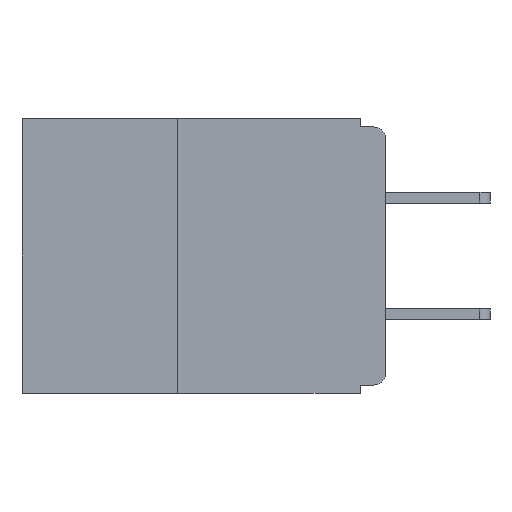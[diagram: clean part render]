
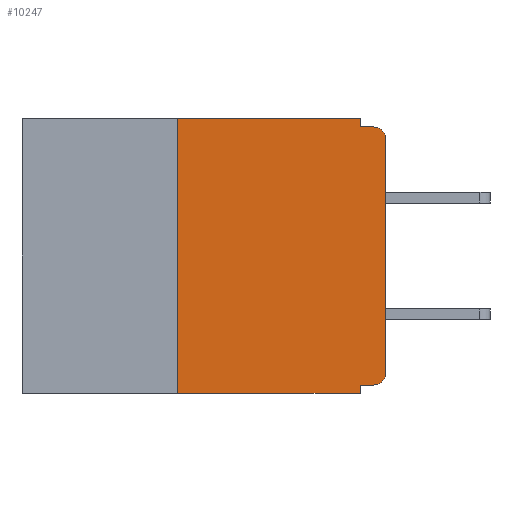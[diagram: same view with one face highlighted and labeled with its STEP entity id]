
A CAD part, left-side view. The second image highlights one B-rep face of the part: STEP entity #10247.
In plain terms, the highlighted planar face has unit normal (-1, 0, 0).
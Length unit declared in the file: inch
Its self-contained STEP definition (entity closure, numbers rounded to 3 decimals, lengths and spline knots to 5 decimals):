
#102 = PLANE ( 'NONE',  #8327 ) ;
#334 = LINE ( 'NONE', #4400, #4716 ) ;
#360 = VERTEX_POINT ( 'NONE', #9620 ) ;
#383 = DIRECTION ( 'NONE',  ( -1., 0., 0. ) ) ;
#410 = ORIENTED_EDGE ( 'NONE', *, *, #1426, .F. ) ;
#419 = ORIENTED_EDGE ( 'NONE', *, *, #1769, .F. ) ;
#715 = CARTESIAN_POINT ( 'NONE',  ( 0., 0., -0.305 ) ) ;
#785 = DIRECTION ( 'NONE',  ( -1., 0., 0. ) ) ;
#812 = CARTESIAN_POINT ( 'NONE',  ( 0., 0.031, -0.01 ) ) ;
#892 = FACE_OUTER_BOUND ( 'NONE', #13292, .T. ) ;
#1267 = VERTEX_POINT ( 'NONE', #11527 ) ;
#1426 = EDGE_CURVE ( 'NONE', #1928, #7709, #1879, .T. ) ;
#1769 = EDGE_CURVE ( 'NONE', #13597, #1928, #334, .T. ) ;
#1823 = ORIENTED_EDGE ( 'NONE', *, *, #1887, .T. ) ;
#1879 = LINE ( 'NONE', #3913, #7350 ) ;
#1887 = EDGE_CURVE ( 'NONE', #3035, #360, #9632, .T. ) ;
#1928 = VERTEX_POINT ( 'NONE', #812 ) ;
#1942 = CARTESIAN_POINT ( 'NONE',  ( 0., 0.015, -0.01 ) ) ;
#2127 = AXIS2_PLACEMENT_3D ( 'NONE', #7322, #785, #8443 ) ;
#2193 = CARTESIAN_POINT ( 'NONE',  ( 0., 0.015, -0.32 ) ) ;
#2365 = VERTEX_POINT ( 'NONE', #11896 ) ;
#2544 = CARTESIAN_POINT ( 'NONE',  ( 0., 0.031, 0. ) ) ;
#3035 = VERTEX_POINT ( 'NONE', #715 ) ;
#3839 = EDGE_CURVE ( 'NONE', #8731, #2365, #7817, .T. ) ;
#3913 = CARTESIAN_POINT ( 'NONE',  ( 0., 0., -0.01 ) ) ;
#4037 = ORIENTED_EDGE ( 'NONE', *, *, #7324, .T. ) ;
#4140 = LINE ( 'NONE', #11265, #6701 ) ;
#4400 = CARTESIAN_POINT ( 'NONE',  ( 0., 0.031, 0. ) ) ;
#4501 = DIRECTION ( 'NONE',  ( 1., 0., 0. ) ) ;
#4716 = VECTOR ( 'NONE', #6992, 39.37008 ) ;
#5465 = VECTOR ( 'NONE', #5669, 39.37008 ) ;
#5535 = DIRECTION ( 'NONE',  ( 0., 0., 1. ) ) ;
#5649 = DIRECTION ( 'NONE',  ( 0., 0., -1. ) ) ;
#5669 = DIRECTION ( 'NONE',  ( 0., -1., 0. ) ) ;
#5678 = CARTESIAN_POINT ( 'NONE',  ( 0., 0.25, -0.33 ) ) ;
#5854 = VERTEX_POINT ( 'NONE', #10892 ) ;
#6592 = EDGE_CURVE ( 'NONE', #5854, #1267, #4140, .T. ) ;
#6701 = VECTOR ( 'NONE', #5649, 39.37008 ) ;
#6922 = CARTESIAN_POINT ( 'NONE',  ( 0., 0.015, -0.025 ) ) ;
#6992 = DIRECTION ( 'NONE',  ( 0., 0., -1. ) ) ;
#7028 = EDGE_CURVE ( 'NONE', #13990, #3035, #10027, .T. ) ;
#7322 = CARTESIAN_POINT ( 'NONE',  ( 0., 0.015, -0.305 ) ) ;
#7324 = EDGE_CURVE ( 'NONE', #8731, #1267, #8412, .T. ) ;
#7350 = VECTOR ( 'NONE', #9466, 39.37008 ) ;
#7709 = VERTEX_POINT ( 'NONE', #1942 ) ;
#7769 = CARTESIAN_POINT ( 'NONE',  ( 0., 0.437, 0. ) ) ;
#7817 = LINE ( 'NONE', #5678, #10489 ) ;
#7854 = CARTESIAN_POINT ( 'NONE',  ( 0., 0.437, -0.33 ) ) ;
#8049 = DIRECTION ( 'NONE',  ( 0., 0., -1. ) ) ;
#8327 = AXIS2_PLACEMENT_3D ( 'NONE', #11185, #4501, #12321 ) ;
#8412 = LINE ( 'NONE', #7854, #5465 ) ;
#8443 = DIRECTION ( 'NONE',  ( 0., 0., -1. ) ) ;
#8454 = EDGE_CURVE ( 'NONE', #2365, #13597, #11133, .T. ) ;
#8731 = VERTEX_POINT ( 'NONE', #12761 ) ;
#8829 = ORIENTED_EDGE ( 'NONE', *, *, #8454, .F. ) ;
#9406 = ORIENTED_EDGE ( 'NONE', *, *, #7028, .T. ) ;
#9466 = DIRECTION ( 'NONE',  ( 0., -1., 0. ) ) ;
#9620 = CARTESIAN_POINT ( 'NONE',  ( 0., 0., -0.025 ) ) ;
#9632 = LINE ( 'NONE', #12699, #12649 ) ;
#9670 = CARTESIAN_POINT ( 'NONE',  ( 0., 0., -0.32 ) ) ;
#9790 = DIRECTION ( 'NONE',  ( 0., 0., 1. ) ) ;
#10027 = CIRCLE ( 'NONE', #2127, 0.015 ) ;
#10055 = ORIENTED_EDGE ( 'NONE', *, *, #3839, .F. ) ;
#10209 = CIRCLE ( 'NONE', #14337, 0.015 ) ;
#10247 = ADVANCED_FACE ( 'NONE', ( #892 ), #102, .F. ) ;
#10386 = EDGE_CURVE ( 'NONE', #360, #7709, #10209, .T. ) ;
#10489 = VECTOR ( 'NONE', #5535, 39.37008 ) ;
#10497 = ORIENTED_EDGE ( 'NONE', *, *, #6592, .F. ) ;
#10712 = ORIENTED_EDGE ( 'NONE', *, *, #13868, .F. ) ;
#10796 = DIRECTION ( 'NONE',  ( 0., 1., 0. ) ) ;
#10892 = CARTESIAN_POINT ( 'NONE',  ( 0., 0.031, -0.32 ) ) ;
#11133 = LINE ( 'NONE', #7769, #13728 ) ;
#11166 = LINE ( 'NONE', #9670, #13761 ) ;
#11185 = CARTESIAN_POINT ( 'NONE',  ( 0., 0.437, 0. ) ) ;
#11265 = CARTESIAN_POINT ( 'NONE',  ( 0., 0.031, -0.33 ) ) ;
#11527 = CARTESIAN_POINT ( 'NONE',  ( 0., 0.031, -0.33 ) ) ;
#11896 = CARTESIAN_POINT ( 'NONE',  ( 0., 0.25, 0. ) ) ;
#12321 = DIRECTION ( 'NONE',  ( 0., 0., -1. ) ) ;
#12649 = VECTOR ( 'NONE', #9790, 39.37008 ) ;
#12699 = CARTESIAN_POINT ( 'NONE',  ( 0., 0., 0. ) ) ;
#12761 = CARTESIAN_POINT ( 'NONE',  ( 0., 0.25, -0.33 ) ) ;
#13292 = EDGE_LOOP ( 'NONE', ( #1823, #14270, #410, #419, #8829, #10055, #4037, #10497, #10712, #9406 ) ) ;
#13430 = DIRECTION ( 'NONE',  ( 0., -1., 0. ) ) ;
#13597 = VERTEX_POINT ( 'NONE', #2544 ) ;
#13728 = VECTOR ( 'NONE', #13430, 39.37008 ) ;
#13761 = VECTOR ( 'NONE', #10796, 39.37008 ) ;
#13868 = EDGE_CURVE ( 'NONE', #13990, #5854, #11166, .T. ) ;
#13990 = VERTEX_POINT ( 'NONE', #2193 ) ;
#14270 = ORIENTED_EDGE ( 'NONE', *, *, #10386, .T. ) ;
#14337 = AXIS2_PLACEMENT_3D ( 'NONE', #6922, #383, #8049 ) ;
